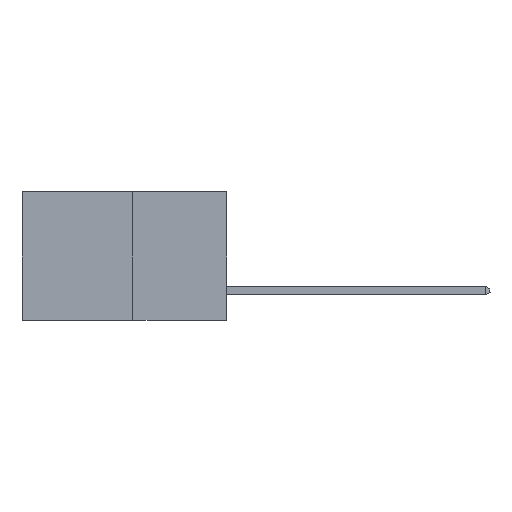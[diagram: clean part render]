
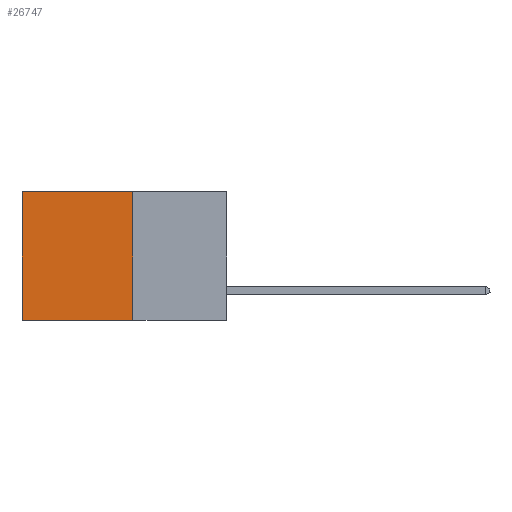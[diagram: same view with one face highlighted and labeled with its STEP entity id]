
A CAD part, left-side view. The second image highlights one B-rep face of the part: STEP entity #26747.
In plain terms, the highlighted planar face has unit normal (-1, 0, 0).
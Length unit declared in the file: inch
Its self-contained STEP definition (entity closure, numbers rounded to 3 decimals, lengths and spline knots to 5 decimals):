
#1159 = DIRECTION ( 'NONE',  ( 1., 0., 0. ) ) ;
#1974 = AXIS2_PLACEMENT_3D ( 'NONE', #25897, #1159, #15720 ) ;
#2719 = VECTOR ( 'NONE', #25031, 39.37008 ) ;
#3604 = EDGE_CURVE ( 'NONE', #4127, #22402, #8232, .T. ) ;
#3647 = CARTESIAN_POINT ( 'NONE',  ( 0.277, 0.27, 0. ) ) ;
#4127 = VERTEX_POINT ( 'NONE', #13931 ) ;
#5309 = FACE_OUTER_BOUND ( 'NONE', #13345, .T. ) ;
#5774 = VECTOR ( 'NONE', #22139, 39.37008 ) ;
#6623 = CARTESIAN_POINT ( 'NONE',  ( 0.277, 0.27, -0.37 ) ) ;
#7167 = EDGE_CURVE ( 'NONE', #15842, #10903, #11292, .T. ) ;
#7358 = LINE ( 'NONE', #24230, #19118 ) ;
#7943 = LINE ( 'NONE', #3647, #12806 ) ;
#8111 = CARTESIAN_POINT ( 'NONE',  ( 0.277, 0.59, 0. ) ) ;
#8232 = LINE ( 'NONE', #25463, #2719 ) ;
#8985 = ORIENTED_EDGE ( 'NONE', *, *, #25587, .T. ) ;
#10567 = ORIENTED_EDGE ( 'NONE', *, *, #24356, .F. ) ;
#10903 = VERTEX_POINT ( 'NONE', #13258 ) ;
#11292 = LINE ( 'NONE', #15972, #5774 ) ;
#11478 = PLANE ( 'NONE',  #1974 ) ;
#12806 = VECTOR ( 'NONE', #16166, 39.37008 ) ;
#13258 = CARTESIAN_POINT ( 'NONE',  ( 0.277, 0.59, -0.37 ) ) ;
#13345 = EDGE_LOOP ( 'NONE', ( #25954, #10567, #21137, #8985 ) ) ;
#13931 = CARTESIAN_POINT ( 'NONE',  ( 0.277, 0.27, 0. ) ) ;
#13981 = DIRECTION ( 'NONE',  ( 0., 1., 0. ) ) ;
#15720 = DIRECTION ( 'NONE',  ( 0., 0., -1. ) ) ;
#15842 = VERTEX_POINT ( 'NONE', #8111 ) ;
#15972 = CARTESIAN_POINT ( 'NONE',  ( 0.277, 0.59, -0.37 ) ) ;
#16166 = DIRECTION ( 'NONE',  ( 0., 1., 0. ) ) ;
#19118 = VECTOR ( 'NONE', #13981, 39.37008 ) ;
#21137 = ORIENTED_EDGE ( 'NONE', *, *, #3604, .F. ) ;
#22139 = DIRECTION ( 'NONE',  ( 0., 0., -1. ) ) ;
#22402 = VERTEX_POINT ( 'NONE', #6623 ) ;
#24230 = CARTESIAN_POINT ( 'NONE',  ( 0.277, 0.27, -0.37 ) ) ;
#24356 = EDGE_CURVE ( 'NONE', #22402, #10903, #7358, .T. ) ;
#25031 = DIRECTION ( 'NONE',  ( 0., 0., -1. ) ) ;
#25463 = CARTESIAN_POINT ( 'NONE',  ( 0.277, 0.27, -0.37 ) ) ;
#25587 = EDGE_CURVE ( 'NONE', #4127, #15842, #7943, .T. ) ;
#25897 = CARTESIAN_POINT ( 'NONE',  ( 0.277, 0.27, -0.37 ) ) ;
#25954 = ORIENTED_EDGE ( 'NONE', *, *, #7167, .T. ) ;
#26747 = ADVANCED_FACE ( 'NONE', ( #5309 ), #11478, .F. ) ;
